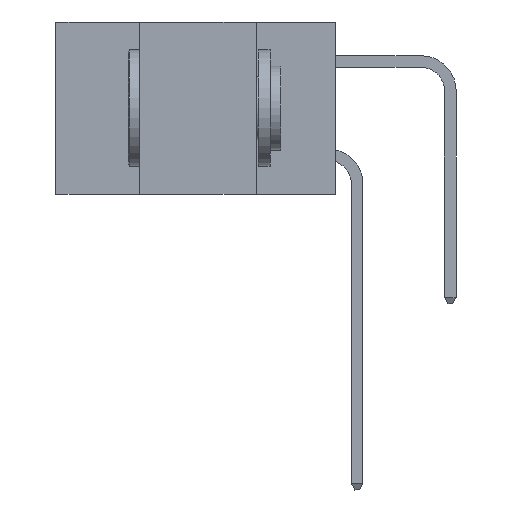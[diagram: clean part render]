
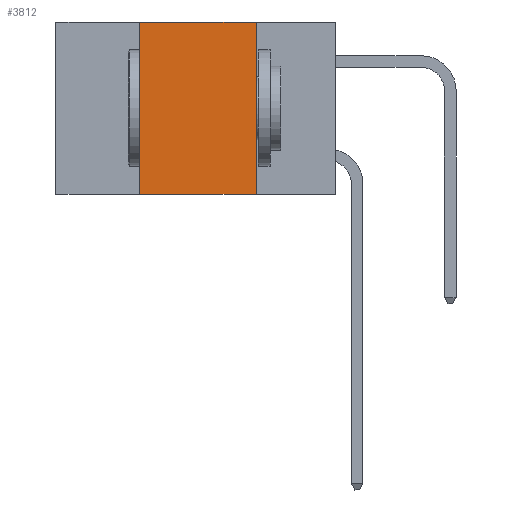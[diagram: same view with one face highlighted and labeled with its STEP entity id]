
A CAD part, left-side view. The second image highlights one B-rep face of the part: STEP entity #3812.
In plain terms, the highlighted planar face has unit normal (-1, 0, 0).
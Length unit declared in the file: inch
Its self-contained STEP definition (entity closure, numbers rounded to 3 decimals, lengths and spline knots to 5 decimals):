
#546 = VERTEX_POINT ( 'NONE', #7363 ) ;
#611 = FACE_OUTER_BOUND ( 'NONE', #8011, .T. ) ;
#954 = ORIENTED_EDGE ( 'NONE', *, *, #10095, .F. ) ;
#1228 = EDGE_CURVE ( 'NONE', #546, #8844, #7609, .T. ) ;
#1965 = CARTESIAN_POINT ( 'NONE',  ( 0., 0.6, 0. ) ) ;
#3054 = LINE ( 'NONE', #3362, #9134 ) ;
#3166 = CARTESIAN_POINT ( 'NONE',  ( 0., 0.17, 0. ) ) ;
#3362 = CARTESIAN_POINT ( 'NONE',  ( 0., 0.42, 0. ) ) ;
#3812 = ADVANCED_FACE ( 'NONE', ( #611 ), #11219, .F. ) ;
#4092 = CARTESIAN_POINT ( 'NONE',  ( 0., 0.6, 0. ) ) ;
#4582 = AXIS2_PLACEMENT_3D ( 'NONE', #1965, #4784, #6589 ) ;
#4784 = DIRECTION ( 'NONE',  ( 1., 0., 0. ) ) ;
#5293 = VECTOR ( 'NONE', #7864, 39.37008 ) ;
#5893 = VECTOR ( 'NONE', #10811, 39.37008 ) ;
#6018 = DIRECTION ( 'NONE',  ( 0., 0., 1. ) ) ;
#6130 = EDGE_CURVE ( 'NONE', #8235, #10253, #6170, .T. ) ;
#6170 = LINE ( 'NONE', #9753, #5893 ) ;
#6450 = ORIENTED_EDGE ( 'NONE', *, *, #6130, .T. ) ;
#6589 = DIRECTION ( 'NONE',  ( 0., 0., -1. ) ) ;
#6616 = CARTESIAN_POINT ( 'NONE',  ( 0., 0.17, 0. ) ) ;
#6991 = DIRECTION ( 'NONE',  ( 0., 0., -1. ) ) ;
#7245 = CARTESIAN_POINT ( 'NONE',  ( 0., 0.17, -0.37 ) ) ;
#7363 = CARTESIAN_POINT ( 'NONE',  ( 0., 0.42, 0. ) ) ;
#7609 = LINE ( 'NONE', #4092, #5293 ) ;
#7864 = DIRECTION ( 'NONE',  ( 0., -1., 0. ) ) ;
#8011 = EDGE_LOOP ( 'NONE', ( #11135, #9659, #954, #6450 ) ) ;
#8235 = VERTEX_POINT ( 'NONE', #10653 ) ;
#8541 = VECTOR ( 'NONE', #6991, 39.37008 ) ;
#8844 = VERTEX_POINT ( 'NONE', #3166 ) ;
#9134 = VECTOR ( 'NONE', #6018, 39.37008 ) ;
#9659 = ORIENTED_EDGE ( 'NONE', *, *, #1228, .F. ) ;
#9753 = CARTESIAN_POINT ( 'NONE',  ( 0., 0.6, -0.37 ) ) ;
#9844 = EDGE_CURVE ( 'NONE', #8844, #10253, #9874, .T. ) ;
#9874 = LINE ( 'NONE', #6616, #8541 ) ;
#10095 = EDGE_CURVE ( 'NONE', #8235, #546, #3054, .T. ) ;
#10253 = VERTEX_POINT ( 'NONE', #7245 ) ;
#10653 = CARTESIAN_POINT ( 'NONE',  ( 0., 0.42, -0.37 ) ) ;
#10811 = DIRECTION ( 'NONE',  ( 0., -1., 0. ) ) ;
#11135 = ORIENTED_EDGE ( 'NONE', *, *, #9844, .F. ) ;
#11219 = PLANE ( 'NONE',  #4582 ) ;
